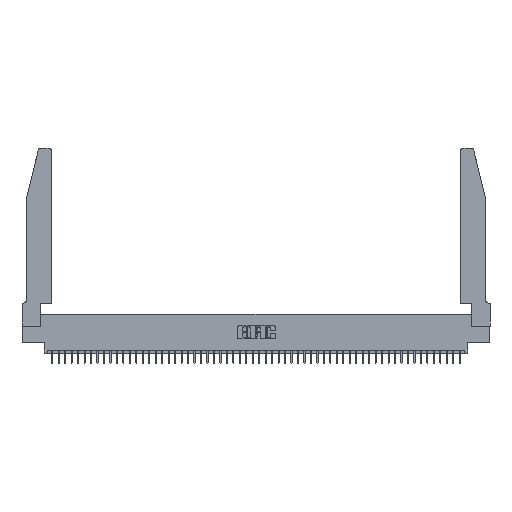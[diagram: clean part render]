
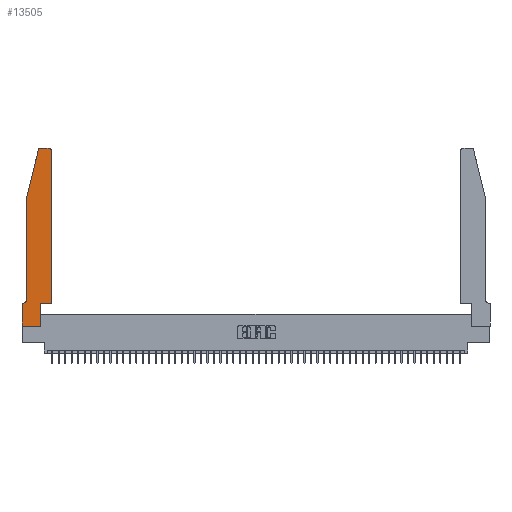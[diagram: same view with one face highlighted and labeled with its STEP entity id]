
A CAD part, top view. The second image highlights one B-rep face of the part: STEP entity #13505.
In plain terms, the highlighted planar face has unit normal (0, 0, 1).
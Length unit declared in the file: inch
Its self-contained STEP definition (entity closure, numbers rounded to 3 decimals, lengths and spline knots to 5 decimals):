
#21 = EDGE_CURVE ( 'NONE', #39710, #10764, #9234, .T. ) ;
#192 = EDGE_CURVE ( 'NONE', #51219, #27185, #44476, .T. ) ;
#468 = CARTESIAN_POINT ( 'NONE',  ( 0.284, 2.75, 0.37 ) ) ;
#787 = ORIENTED_EDGE ( 'NONE', *, *, #15474, .T. ) ;
#1003 = ORIENTED_EDGE ( 'NONE', *, *, #7809, .T. ) ;
#1037 = LINE ( 'NONE', #37717, #43995 ) ;
#1535 = CIRCLE ( 'NONE', #19119, 0.03 ) ;
#1583 = DIRECTION ( 'NONE',  ( 1., 0., 0. ) ) ;
#1860 = VERTEX_POINT ( 'NONE', #49161 ) ;
#2136 = CARTESIAN_POINT ( 'NONE',  ( 0., 0., 0.37 ) ) ;
#3427 = CARTESIAN_POINT ( 'NONE',  ( 0.4505, 0.35, 0.37 ) ) ;
#4353 = VERTEX_POINT ( 'NONE', #51459 ) ;
#6091 = ORIENTED_EDGE ( 'NONE', *, *, #21, .T. ) ;
#6886 = DIRECTION ( 'NONE',  ( 0., -1., 0. ) ) ;
#7686 = CARTESIAN_POINT ( 'NONE',  ( 0.4205, 2.75, 0.37 ) ) ;
#7809 = EDGE_CURVE ( 'NONE', #37053, #18731, #30043, .T. ) ;
#7978 = VECTOR ( 'NONE', #6886, 39.37008 ) ;
#8185 = EDGE_CURVE ( 'NONE', #25963, #4353, #1535, .T. ) ;
#9234 = LINE ( 'NONE', #47151, #7978 ) ;
#9276 = LINE ( 'NONE', #19409, #10529 ) ;
#9661 = EDGE_CURVE ( 'NONE', #18731, #51219, #9276, .T. ) ;
#9681 = ORIENTED_EDGE ( 'NONE', *, *, #42325, .T. ) ;
#10529 = VECTOR ( 'NONE', #35351, 39.37008 ) ;
#10764 = VERTEX_POINT ( 'NONE', #2136 ) ;
#10948 = ORIENTED_EDGE ( 'NONE', *, *, #8185, .T. ) ;
#11127 = VECTOR ( 'NONE', #19925, 39.37008 ) ;
#11149 = CARTESIAN_POINT ( 'NONE',  ( 0.2865, 0.35, 0.37 ) ) ;
#13505 = ADVANCED_FACE ( 'NONE', ( #29096 ), #17522, .T. ) ;
#13608 = DIRECTION ( 'NONE',  ( 0., -1., 0. ) ) ;
#13793 = VERTEX_POINT ( 'NONE', #43303 ) ;
#13968 = CARTESIAN_POINT ( 'NONE',  ( 0.2865, 0.35, 0.37 ) ) ;
#14129 = ORIENTED_EDGE ( 'NONE', *, *, #24012, .T. ) ;
#14380 = ORIENTED_EDGE ( 'NONE', *, *, #32838, .T. ) ;
#15161 = CARTESIAN_POINT ( 'NONE',  ( 0., 0.35, 0.37 ) ) ;
#15302 = LINE ( 'NONE', #11149, #35407 ) ;
#15474 = EDGE_CURVE ( 'NONE', #1860, #26673, #1037, .T. ) ;
#15660 = ORIENTED_EDGE ( 'NONE', *, *, #192, .T. ) ;
#16355 = DIRECTION ( 'NONE',  ( -1., 0., 0. ) ) ;
#17522 = PLANE ( 'NONE',  #34398 ) ;
#17995 = CIRCLE ( 'NONE', #43114, 0.07 ) ;
#18271 = VECTOR ( 'NONE', #37635, 39.37008 ) ;
#18731 = VERTEX_POINT ( 'NONE', #31350 ) ;
#19119 = AXIS2_PLACEMENT_3D ( 'NONE', #49874, #25829, #1583 ) ;
#19409 = CARTESIAN_POINT ( 'NONE',  ( 0.4505, 0.35, 0.37 ) ) ;
#19500 = AXIS2_PLACEMENT_3D ( 'NONE', #44036, #19969, #48027 ) ;
#19542 = LINE ( 'NONE', #45535, #18271 ) ;
#19925 = DIRECTION ( 'NONE',  ( 1., 0., 0. ) ) ;
#19969 = DIRECTION ( 'NONE',  ( 0., 0., 1. ) ) ;
#20667 = ORIENTED_EDGE ( 'NONE', *, *, #52109, .T. ) ;
#21536 = CARTESIAN_POINT ( 'NONE',  ( 0., 0.35, 0.37 ) ) ;
#22056 = DIRECTION ( 'NONE',  ( -1., 0., 0. ) ) ;
#22928 = CARTESIAN_POINT ( 'NONE',  ( 0.0055, 0.42, 0.37 ) ) ;
#23148 = CARTESIAN_POINT ( 'NONE',  ( 0.4505, 2.72, 0.37 ) ) ;
#23323 = DIRECTION ( 'NONE',  ( 0., 1., 0. ) ) ;
#24012 = EDGE_CURVE ( 'NONE', #26673, #30767, #17995, .T. ) ;
#24468 = LINE ( 'NONE', #40427, #35106 ) ;
#25577 = DIRECTION ( 'NONE',  ( 1., 0., 0. ) ) ;
#25829 = DIRECTION ( 'NONE',  ( 0., 0., 1. ) ) ;
#25963 = VERTEX_POINT ( 'NONE', #468 ) ;
#26673 = VERTEX_POINT ( 'NONE', #32894 ) ;
#26862 = LINE ( 'NONE', #38058, #46944 ) ;
#26947 = DIRECTION ( 'NONE',  ( -1., 0., 0. ) ) ;
#27185 = VERTEX_POINT ( 'NONE', #7686 ) ;
#29096 = FACE_OUTER_BOUND ( 'NONE', #33305, .T. ) ;
#29446 = EDGE_CURVE ( 'NONE', #13793, #37053, #15302, .T. ) ;
#30043 = LINE ( 'NONE', #3427, #39493 ) ;
#30767 = VERTEX_POINT ( 'NONE', #48285 ) ;
#31350 = CARTESIAN_POINT ( 'NONE',  ( 0.4505, 0.35, 0.37 ) ) ;
#32350 = ORIENTED_EDGE ( 'NONE', *, *, #50268, .T. ) ;
#32838 = EDGE_CURVE ( 'NONE', #30767, #39710, #24468, .T. ) ;
#32894 = CARTESIAN_POINT ( 'NONE',  ( 0.0755, 0.42, 0.37 ) ) ;
#33227 = ORIENTED_EDGE ( 'NONE', *, *, #9661, .T. ) ;
#33305 = EDGE_LOOP ( 'NONE', ( #9681, #10948, #32350, #787, #14129, #14380, #6091, #20667, #44557, #1003, #33227, #15660 ) ) ;
#33757 = LINE ( 'NONE', #39946, #11127 ) ;
#34398 = AXIS2_PLACEMENT_3D ( 'NONE', #21536, #49624, #25577 ) ;
#35106 = VECTOR ( 'NONE', #16355, 39.37008 ) ;
#35351 = DIRECTION ( 'NONE',  ( 0., 1., 0. ) ) ;
#35407 = VECTOR ( 'NONE', #23323, 39.37008 ) ;
#37053 = VERTEX_POINT ( 'NONE', #13968 ) ;
#37635 = DIRECTION ( 'NONE',  ( -0.239, -0.971, 0. ) ) ;
#37717 = CARTESIAN_POINT ( 'NONE',  ( 0.0755, 2., 0.37 ) ) ;
#38058 = CARTESIAN_POINT ( 'NONE',  ( 0.2605, 2.75, 0.37 ) ) ;
#39493 = VECTOR ( 'NONE', #39756, 39.37008 ) ;
#39710 = VERTEX_POINT ( 'NONE', #15161 ) ;
#39756 = DIRECTION ( 'NONE',  ( 1., 0., 0. ) ) ;
#39946 = CARTESIAN_POINT ( 'NONE',  ( 0., 0., 0.37 ) ) ;
#40427 = CARTESIAN_POINT ( 'NONE',  ( 0.0755, 0.35, 0.37 ) ) ;
#42325 = EDGE_CURVE ( 'NONE', #27185, #25963, #26862, .T. ) ;
#43114 = AXIS2_PLACEMENT_3D ( 'NONE', #22928, #51007, #26947 ) ;
#43303 = CARTESIAN_POINT ( 'NONE',  ( 0.2865, 0., 0.37 ) ) ;
#43995 = VECTOR ( 'NONE', #13608, 39.37008 ) ;
#44036 = CARTESIAN_POINT ( 'NONE',  ( 0.4205, 2.72, 0.37 ) ) ;
#44476 = CIRCLE ( 'NONE', #19500, 0.03 ) ;
#44557 = ORIENTED_EDGE ( 'NONE', *, *, #29446, .T. ) ;
#45535 = CARTESIAN_POINT ( 'NONE',  ( 0.0755, 2., 0.37 ) ) ;
#46944 = VECTOR ( 'NONE', #22056, 39.37008 ) ;
#47151 = CARTESIAN_POINT ( 'NONE',  ( 0., 0., 0.37 ) ) ;
#48027 = DIRECTION ( 'NONE',  ( 1., 0., 0. ) ) ;
#48285 = CARTESIAN_POINT ( 'NONE',  ( 0.0055, 0.35, 0.37 ) ) ;
#49161 = CARTESIAN_POINT ( 'NONE',  ( 0.0755, 2., 0.37 ) ) ;
#49624 = DIRECTION ( 'NONE',  ( 0., 0., 1. ) ) ;
#49874 = CARTESIAN_POINT ( 'NONE',  ( 0.284, 2.72, 0.37 ) ) ;
#50268 = EDGE_CURVE ( 'NONE', #4353, #1860, #19542, .T. ) ;
#51007 = DIRECTION ( 'NONE',  ( 0., 0., -1. ) ) ;
#51219 = VERTEX_POINT ( 'NONE', #23148 ) ;
#51459 = CARTESIAN_POINT ( 'NONE',  ( 0.25487, 2.72718, 0.37 ) ) ;
#52109 = EDGE_CURVE ( 'NONE', #10764, #13793, #33757, .T. ) ;
